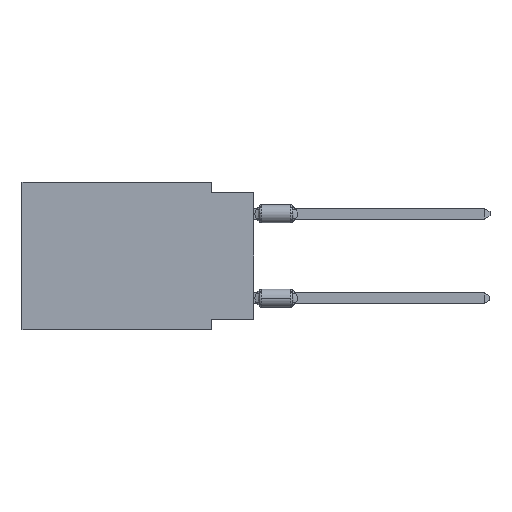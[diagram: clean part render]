
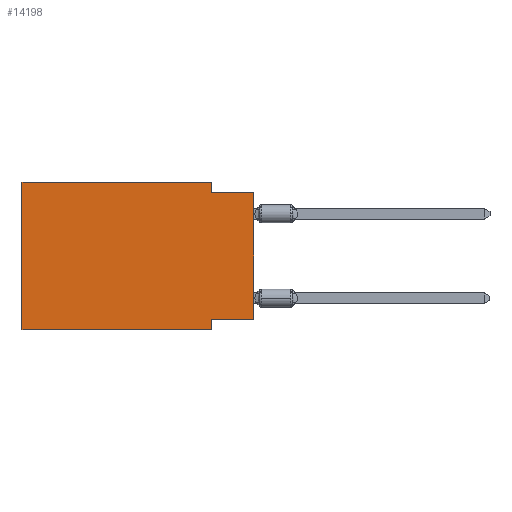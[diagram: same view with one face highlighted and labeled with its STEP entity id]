
A CAD part, left-side view. The second image highlights one B-rep face of the part: STEP entity #14198.
In plain terms, the highlighted planar face has unit normal (-1, 0, 0).
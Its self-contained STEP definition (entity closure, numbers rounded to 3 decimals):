
#44 = ORIENTED_EDGE ( 'NONE', *, *, #13951, .F. ) ;
#162 = LINE ( 'NONE', #14562, #15826 ) ;
#589 = CARTESIAN_POINT ( 'NONE',  ( 0., 2.54, 0. ) ) ;
#975 = DIRECTION ( 'NONE',  ( 0., 0., 1. ) ) ;
#1027 = LINE ( 'NONE', #11201, #13127 ) ;
#1135 = EDGE_CURVE ( 'NONE', #8522, #1663, #11666, .T. ) ;
#1339 = LINE ( 'NONE', #8020, #2348 ) ;
#1457 = CARTESIAN_POINT ( 'NONE',  ( 0., 0., 0. ) ) ;
#1663 = VERTEX_POINT ( 'NONE', #13076 ) ;
#2348 = VECTOR ( 'NONE', #14123, 1000. ) ;
#2593 = AXIS2_PLACEMENT_3D ( 'NONE', #16236, #12357, #13373 ) ;
#3127 = VERTEX_POINT ( 'NONE', #8100 ) ;
#3175 = CARTESIAN_POINT ( 'NONE',  ( 0., 2.54, -0.635 ) ) ;
#3201 = VECTOR ( 'NONE', #5532, 1000. ) ;
#3450 = EDGE_CURVE ( 'NONE', #11459, #8522, #10375, .T. ) ;
#3516 = EDGE_LOOP ( 'NONE', ( #13365, #44, #13997, #14224, #14998, #8019, #11429, #6854 ) ) ;
#3867 = CARTESIAN_POINT ( 'NONE',  ( 0., 2.54, -8.89 ) ) ;
#3874 = EDGE_CURVE ( 'NONE', #14407, #1663, #1027, .T. ) ;
#4564 = FACE_OUTER_BOUND ( 'NONE', #3516, .T. ) ;
#5532 = DIRECTION ( 'NONE',  ( 0., 0., -1. ) ) ;
#5687 = EDGE_CURVE ( 'NONE', #9346, #13740, #162, .T. ) ;
#5915 = CARTESIAN_POINT ( 'NONE',  ( 0., 13.97, 0. ) ) ;
#6177 = CARTESIAN_POINT ( 'NONE',  ( 0., 0., -8.255 ) ) ;
#6854 = ORIENTED_EDGE ( 'NONE', *, *, #3450, .F. ) ;
#7049 = EDGE_CURVE ( 'NONE', #14407, #9346, #13945, .T. ) ;
#7339 = VERTEX_POINT ( 'NONE', #3175 ) ;
#8019 = ORIENTED_EDGE ( 'NONE', *, *, #3874, .T. ) ;
#8020 = CARTESIAN_POINT ( 'NONE',  ( 0., 0., -0.635 ) ) ;
#8100 = CARTESIAN_POINT ( 'NONE',  ( 0., 0., -0.635 ) ) ;
#8193 = PLANE ( 'NONE',  #2593 ) ;
#8214 = CARTESIAN_POINT ( 'NONE',  ( 0., 13.97, 0. ) ) ;
#8522 = VERTEX_POINT ( 'NONE', #13031 ) ;
#8677 = DIRECTION ( 'NONE',  ( 0., 1., 0. ) ) ;
#8999 = DIRECTION ( 'NONE',  ( 0., 0., 1. ) ) ;
#9253 = CARTESIAN_POINT ( 'NONE',  ( 0., 2.54, 0. ) ) ;
#9346 = VERTEX_POINT ( 'NONE', #8214 ) ;
#10375 = LINE ( 'NONE', #15443, #13660 ) ;
#10458 = VECTOR ( 'NONE', #8999, 1000. ) ;
#11201 = CARTESIAN_POINT ( 'NONE',  ( 0., 13.97, -8.89 ) ) ;
#11429 = ORIENTED_EDGE ( 'NONE', *, *, #1135, .F. ) ;
#11459 = VERTEX_POINT ( 'NONE', #6177 ) ;
#11639 = LINE ( 'NONE', #1457, #10458 ) ;
#11666 = LINE ( 'NONE', #3867, #14902 ) ;
#11972 = LINE ( 'NONE', #9253, #3201 ) ;
#12357 = DIRECTION ( 'NONE',  ( 1., 0., 0. ) ) ;
#12558 = DIRECTION ( 'NONE',  ( 0., -1., 0. ) ) ;
#13031 = CARTESIAN_POINT ( 'NONE',  ( 0., 2.54, -8.255 ) ) ;
#13076 = CARTESIAN_POINT ( 'NONE',  ( 0., 2.54, -8.89 ) ) ;
#13127 = VECTOR ( 'NONE', #12558, 1000. ) ;
#13220 = DIRECTION ( 'NONE',  ( 0., -1., 0. ) ) ;
#13365 = ORIENTED_EDGE ( 'NONE', *, *, #13535, .T. ) ;
#13373 = DIRECTION ( 'NONE',  ( 0., 0., -1. ) ) ;
#13535 = EDGE_CURVE ( 'NONE', #11459, #3127, #11639, .T. ) ;
#13660 = VECTOR ( 'NONE', #8677, 1000. ) ;
#13740 = VERTEX_POINT ( 'NONE', #589 ) ;
#13945 = LINE ( 'NONE', #5915, #14940 ) ;
#13951 = EDGE_CURVE ( 'NONE', #7339, #3127, #1339, .T. ) ;
#13997 = ORIENTED_EDGE ( 'NONE', *, *, #15182, .F. ) ;
#14123 = DIRECTION ( 'NONE',  ( 0., -1., 0. ) ) ;
#14198 = ADVANCED_FACE ( 'NONE', ( #4564 ), #8193, .F. ) ;
#14224 = ORIENTED_EDGE ( 'NONE', *, *, #5687, .F. ) ;
#14407 = VERTEX_POINT ( 'NONE', #15710 ) ;
#14562 = CARTESIAN_POINT ( 'NONE',  ( 0., 13.97, 0. ) ) ;
#14902 = VECTOR ( 'NONE', #15460, 1000. ) ;
#14940 = VECTOR ( 'NONE', #975, 1000. ) ;
#14998 = ORIENTED_EDGE ( 'NONE', *, *, #7049, .F. ) ;
#15182 = EDGE_CURVE ( 'NONE', #13740, #7339, #11972, .T. ) ;
#15443 = CARTESIAN_POINT ( 'NONE',  ( 0., 0., -8.255 ) ) ;
#15460 = DIRECTION ( 'NONE',  ( 0., 0., -1. ) ) ;
#15710 = CARTESIAN_POINT ( 'NONE',  ( 0., 13.97, -8.89 ) ) ;
#15826 = VECTOR ( 'NONE', #13220, 1000. ) ;
#16236 = CARTESIAN_POINT ( 'NONE',  ( 0., 13.97, 0. ) ) ;
